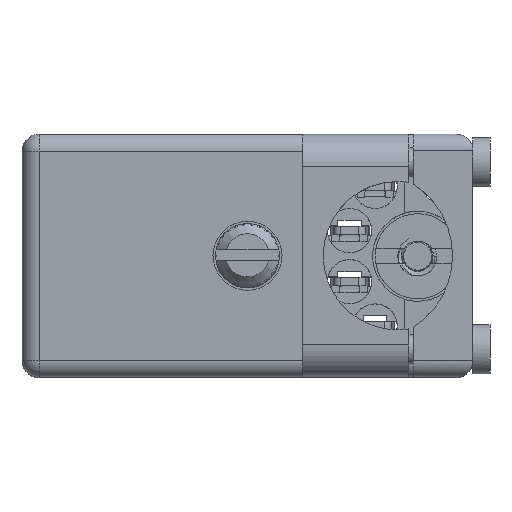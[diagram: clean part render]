
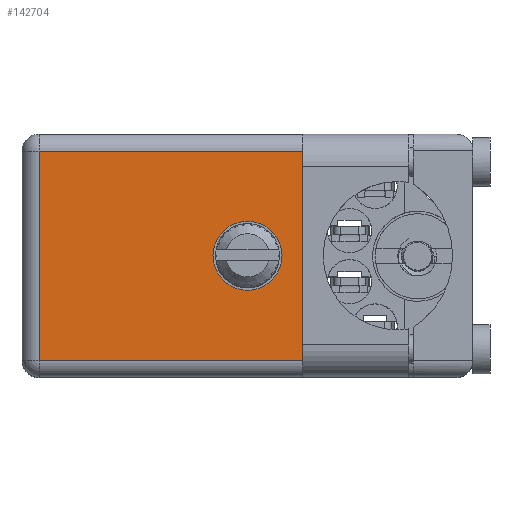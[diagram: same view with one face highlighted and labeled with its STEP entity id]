
A CAD part, top view. The second image highlights one B-rep face of the part: STEP entity #142704.
In plain terms, the highlighted face is planar.
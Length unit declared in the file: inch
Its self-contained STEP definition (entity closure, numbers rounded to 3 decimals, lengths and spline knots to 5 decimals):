
#4692 = ORIENTED_EDGE ( 'NONE', *, *, #81810, .F. ) ;
#5732 = CARTESIAN_POINT ( 'NONE',  ( 0.4875, 0.806, 0.245 ) ) ;
#17206 = EDGE_LOOP ( 'NONE', ( #4692, #110066 ) ) ;
#20184 = ORIENTED_EDGE ( 'NONE', *, *, #161133, .T. ) ;
#20421 = LINE ( 'NONE', #123754, #109446 ) ;
#22634 = CARTESIAN_POINT ( 'NONE',  ( 0.2025, 0.806, 0.245 ) ) ;
#26897 = CARTESIAN_POINT ( 'NONE',  ( 0.2025, 0.806, -0.245 ) ) ;
#29359 = AXIS2_PLACEMENT_3D ( 'NONE', #61027, #121002, #60375 ) ;
#31639 = CIRCLE ( 'NONE', #29359, 0.1015 ) ;
#34040 = CARTESIAN_POINT ( 'NONE',  ( 0.2025, 0.806, 0.245 ) ) ;
#36447 = CARTESIAN_POINT ( 'NONE',  ( -0.6625, 0.806, -0.3075 ) ) ;
#40342 = DIRECTION ( 'NONE',  ( 0., 1., 0. ) ) ;
#41330 = DIRECTION ( 'NONE',  ( 0., 1., 0. ) ) ;
#42142 = EDGE_CURVE ( 'NONE', #199809, #198212, #196328, .T. ) ;
#42860 = EDGE_CURVE ( 'NONE', #178813, #180419, #20421, .T. ) ;
#46742 = EDGE_CURVE ( 'NONE', #144688, #89971, #31639, .T. ) ;
#50582 = ORIENTED_EDGE ( 'NONE', *, *, #93816, .T. ) ;
#60375 = DIRECTION ( 'NONE',  ( 0., 0., 1. ) ) ;
#60467 = CARTESIAN_POINT ( 'NONE',  ( 0.4875, 0.806, -0.245 ) ) ;
#61027 = CARTESIAN_POINT ( 'NONE',  ( 0., 0.806, 0. ) ) ;
#61858 = FACE_OUTER_BOUND ( 'NONE', #157681, .T. ) ;
#62321 = ORIENTED_EDGE ( 'NONE', *, *, #182339, .T. ) ;
#64149 = ORIENTED_EDGE ( 'NONE', *, *, #42860, .F. ) ;
#64939 = DIRECTION ( 'NONE',  ( 0., 0., -1. ) ) ;
#69910 = LINE ( 'NONE', #26897, #142192 ) ;
#74700 = CARTESIAN_POINT ( 'NONE',  ( 0.2025, 0.806, -0.245 ) ) ;
#81810 = EDGE_CURVE ( 'NONE', #89971, #144688, #199148, .T. ) ;
#87409 = CARTESIAN_POINT ( 'NONE',  ( 0., 0.806, 0. ) ) ;
#87415 = DIRECTION ( 'NONE',  ( 1., 0., 0. ) ) ;
#89971 = VERTEX_POINT ( 'NONE', #122724 ) ;
#93816 = EDGE_CURVE ( 'NONE', #138265, #152692, #69910, .T. ) ;
#96061 = DIRECTION ( 'NONE',  ( 0., 0., 1. ) ) ;
#96416 = VERTEX_POINT ( 'NONE', #163313 ) ;
#98487 = LINE ( 'NONE', #140221, #149104 ) ;
#98547 = AXIS2_PLACEMENT_3D ( 'NONE', #87409, #40342, #162858 ) ;
#101897 = DIRECTION ( 'NONE',  ( -1., 0., 0. ) ) ;
#102642 = VERTEX_POINT ( 'NONE', #193448 ) ;
#103163 = EDGE_CURVE ( 'NONE', #96416, #138265, #187737, .T. ) ;
#109098 = CARTESIAN_POINT ( 'NONE',  ( 0.4875, 0.806, -0.3075 ) ) ;
#109446 = VECTOR ( 'NONE', #96061, 39.37008 ) ;
#110066 = ORIENTED_EDGE ( 'NONE', *, *, #46742, .F. ) ;
#113337 = CARTESIAN_POINT ( 'NONE',  ( 0.4875, 0.806, 0.3075 ) ) ;
#113344 = VECTOR ( 'NONE', #126834, 39.37008 ) ;
#115456 = VECTOR ( 'NONE', #64939, 39.37008 ) ;
#121002 = DIRECTION ( 'NONE',  ( 0., 1., 0. ) ) ;
#121067 = VECTOR ( 'NONE', #145949, 39.37008 ) ;
#122724 = CARTESIAN_POINT ( 'NONE',  ( 0., 0.806, 0.1015 ) ) ;
#123754 = CARTESIAN_POINT ( 'NONE',  ( 0.4875, 0.806, -0.3575 ) ) ;
#126834 = DIRECTION ( 'NONE',  ( 1., 0., 0. ) ) ;
#130316 = DIRECTION ( 'NONE',  ( -1., 0., 0. ) ) ;
#134211 = CARTESIAN_POINT ( 'NONE',  ( -0.6625, 0.806, -0.3575 ) ) ;
#136658 = FACE_BOUND ( 'NONE', #17206, .T. ) ;
#138265 = VERTEX_POINT ( 'NONE', #74700 ) ;
#139666 = VECTOR ( 'NONE', #130316, 39.37008 ) ;
#140221 = CARTESIAN_POINT ( 'NONE',  ( 0.4875, 0.806, -0.3575 ) ) ;
#142192 = VECTOR ( 'NONE', #87415, 39.37008 ) ;
#142704 = ADVANCED_FACE ( 'NONE', ( #61858, #136658 ), #162524, .T. ) ;
#144688 = VERTEX_POINT ( 'NONE', #154785 ) ;
#145914 = ORIENTED_EDGE ( 'NONE', *, *, #161751, .F. ) ;
#145949 = DIRECTION ( 'NONE',  ( 0., 0., 1. ) ) ;
#147365 = AXIS2_PLACEMENT_3D ( 'NONE', #134211, #41330, #101897 ) ;
#149104 = VECTOR ( 'NONE', #154406, 39.37008 ) ;
#152692 = VERTEX_POINT ( 'NONE', #60467 ) ;
#154291 = LINE ( 'NONE', #113337, #113344 ) ;
#154406 = DIRECTION ( 'NONE',  ( 0., 0., 1. ) ) ;
#154785 = CARTESIAN_POINT ( 'NONE',  ( 0., 0.806, -0.1015 ) ) ;
#156497 = LINE ( 'NONE', #22634, #139666 ) ;
#157681 = EDGE_LOOP ( 'NONE', ( #62321, #195964, #64149, #20184, #190297, #50582, #145914, #190533 ) ) ;
#161133 = EDGE_CURVE ( 'NONE', #178813, #96416, #156497, .T. ) ;
#161751 = EDGE_CURVE ( 'NONE', #199809, #152692, #98487, .T. ) ;
#161965 = LINE ( 'NONE', #178273, #121067 ) ;
#162524 = PLANE ( 'NONE',  #147365 ) ;
#162858 = DIRECTION ( 'NONE',  ( 0., 0., 1. ) ) ;
#163313 = CARTESIAN_POINT ( 'NONE',  ( 0.2025, 0.806, 0.245 ) ) ;
#166219 = CARTESIAN_POINT ( 'NONE',  ( 0.4875, 0.806, 0.3075 ) ) ;
#178273 = CARTESIAN_POINT ( 'NONE',  ( -0.6125, 0.806, -0.3575 ) ) ;
#178813 = VERTEX_POINT ( 'NONE', #5732 ) ;
#180419 = VERTEX_POINT ( 'NONE', #166219 ) ;
#182339 = EDGE_CURVE ( 'NONE', #198212, #102642, #161965, .T. ) ;
#185227 = EDGE_CURVE ( 'NONE', #102642, #180419, #154291, .T. ) ;
#186736 = VECTOR ( 'NONE', #189264, 39.37008 ) ;
#187737 = LINE ( 'NONE', #34040, #115456 ) ;
#189264 = DIRECTION ( 'NONE',  ( -1., 0., 0. ) ) ;
#190297 = ORIENTED_EDGE ( 'NONE', *, *, #103163, .T. ) ;
#190533 = ORIENTED_EDGE ( 'NONE', *, *, #42142, .T. ) ;
#193448 = CARTESIAN_POINT ( 'NONE',  ( -0.6125, 0.806, 0.3075 ) ) ;
#193788 = CARTESIAN_POINT ( 'NONE',  ( -0.6125, 0.806, -0.3075 ) ) ;
#195964 = ORIENTED_EDGE ( 'NONE', *, *, #185227, .T. ) ;
#196328 = LINE ( 'NONE', #36447, #186736 ) ;
#198212 = VERTEX_POINT ( 'NONE', #193788 ) ;
#199148 = CIRCLE ( 'NONE', #98547, 0.1015 ) ;
#199809 = VERTEX_POINT ( 'NONE', #109098 ) ;
